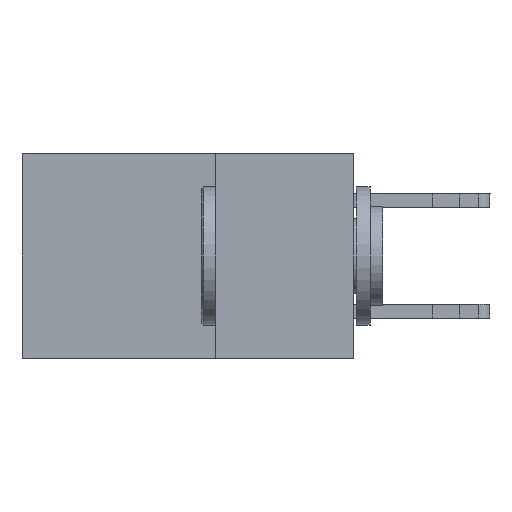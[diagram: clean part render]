
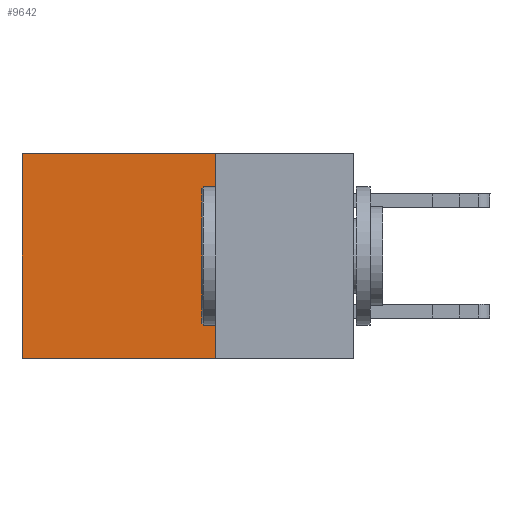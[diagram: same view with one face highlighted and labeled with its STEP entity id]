
A CAD part, left-side view. The second image highlights one B-rep face of the part: STEP entity #9642.
In plain terms, the highlighted planar face has unit normal (-1, 0, 0).
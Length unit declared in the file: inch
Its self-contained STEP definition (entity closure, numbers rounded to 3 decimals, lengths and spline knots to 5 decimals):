
#431 = CARTESIAN_POINT ( 'NONE',  ( 0.2875, 0.6, 0. ) ) ;
#463 = ORIENTED_EDGE ( 'NONE', *, *, #16174, .T. ) ;
#753 = CARTESIAN_POINT ( 'NONE',  ( 0.2875, 0.25, 0. ) ) ;
#2319 = CARTESIAN_POINT ( 'NONE',  ( 0.2875, 0.25, 0. ) ) ;
#5643 = PLANE ( 'NONE',  #28102 ) ;
#5864 = LINE ( 'NONE', #9270, #11506 ) ;
#8418 = VERTEX_POINT ( 'NONE', #26059 ) ;
#9270 = CARTESIAN_POINT ( 'NONE',  ( 0.2875, 0.6, 0. ) ) ;
#9642 = ADVANCED_FACE ( 'NONE', ( #27451 ), #5643, .F. ) ;
#9785 = DIRECTION ( 'NONE',  ( 0., 0., -1. ) ) ;
#10253 = EDGE_CURVE ( 'NONE', #12721, #21828, #18629, .T. ) ;
#11506 = VECTOR ( 'NONE', #20214, 39.37008 ) ;
#11878 = ORIENTED_EDGE ( 'NONE', *, *, #10253, .F. ) ;
#12397 = ORIENTED_EDGE ( 'NONE', *, *, #24684, .F. ) ;
#12721 = VERTEX_POINT ( 'NONE', #16425 ) ;
#14858 = LINE ( 'NONE', #2319, #26065 ) ;
#16174 = EDGE_CURVE ( 'NONE', #18958, #21828, #5864, .T. ) ;
#16425 = CARTESIAN_POINT ( 'NONE',  ( 0.2875, 0.25, -0.37 ) ) ;
#17456 = EDGE_LOOP ( 'NONE', ( #463, #11878, #12397, #23179 ) ) ;
#18429 = CARTESIAN_POINT ( 'NONE',  ( 0.2875, 0.25, -0.37 ) ) ;
#18629 = LINE ( 'NONE', #18429, #20035 ) ;
#18958 = VERTEX_POINT ( 'NONE', #431 ) ;
#20035 = VECTOR ( 'NONE', #25203, 39.37008 ) ;
#20214 = DIRECTION ( 'NONE',  ( 0., 0., -1. ) ) ;
#20431 = DIRECTION ( 'NONE',  ( 0., 0., -1. ) ) ;
#20953 = DIRECTION ( 'NONE',  ( 0., 1., 0. ) ) ;
#21308 = CARTESIAN_POINT ( 'NONE',  ( 0.2875, 0.25, 0. ) ) ;
#21828 = VERTEX_POINT ( 'NONE', #28722 ) ;
#23179 = ORIENTED_EDGE ( 'NONE', *, *, #24211, .T. ) ;
#24211 = EDGE_CURVE ( 'NONE', #8418, #18958, #24330, .T. ) ;
#24330 = LINE ( 'NONE', #753, #26092 ) ;
#24684 = EDGE_CURVE ( 'NONE', #8418, #12721, #14858, .T. ) ;
#25203 = DIRECTION ( 'NONE',  ( 0., 1., 0. ) ) ;
#25530 = DIRECTION ( 'NONE',  ( 1., 0., 0. ) ) ;
#26059 = CARTESIAN_POINT ( 'NONE',  ( 0.2875, 0.25, 0. ) ) ;
#26065 = VECTOR ( 'NONE', #20431, 39.37008 ) ;
#26092 = VECTOR ( 'NONE', #20953, 39.37008 ) ;
#27451 = FACE_OUTER_BOUND ( 'NONE', #17456, .T. ) ;
#28102 = AXIS2_PLACEMENT_3D ( 'NONE', #21308, #25530, #9785 ) ;
#28722 = CARTESIAN_POINT ( 'NONE',  ( 0.2875, 0.6, -0.37 ) ) ;
